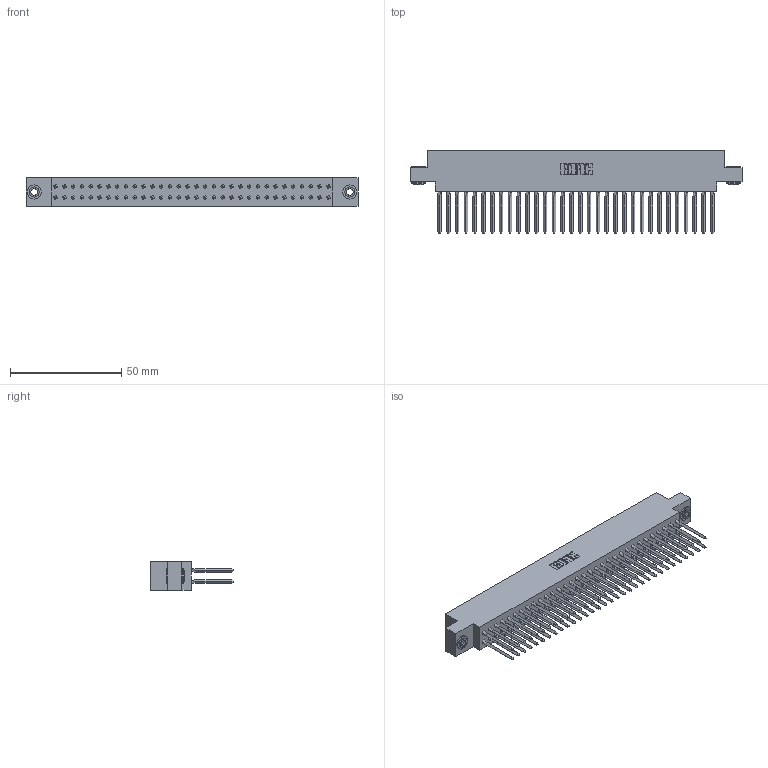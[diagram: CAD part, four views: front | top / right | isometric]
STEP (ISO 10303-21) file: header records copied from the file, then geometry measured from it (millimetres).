
FILE_DESCRIPTION (( 'STEP AP203' ), '1' );
FILE_NAME ('317-064-542-803.STEP', '2020-02-28T05:53:12', ( '' ), ( '' ), 'SwSTEP 2.0', 'SolidWorks 2016', '' );
FILE_SCHEMA (( 'CONFIG_CONTROL_DESIGN' ));
Length unit declared in the file: inch
Products named in the file (4): 345-250-002_345-250-002-102; 317 Part_.156 Dia - TH; 317-290-003_542; 317-064-542-803
Assembly tree (67 placements, depth 2):
  317-064-542-803
    317 Part_.156 Dia - TH
    317-290-003_542  x64
    345-250-002_345-250-002-102  x2
Bounding box: 149.5 x 37.34 x 12.7 mm (x, y, z)
Volume: 24184.2 mm3; surface area: 33525.7 mm2
Topology: 67 solids, 67 shells, 3788 faces, 10591 edges, 6758 vertices
Faces by surface type: plane 3012, cylinder 512, bspline 256, cone 8
Entity records: 47318 total; most frequent: CARTESIAN_POINT 8472, ORIENTED_EDGE 8128, DIRECTION 6894, EDGE_CURVE 4064, VECTOR 3870, LINE 3870, VERTEX_POINT 2702, AXIS2_PLACEMENT_3D 1512
